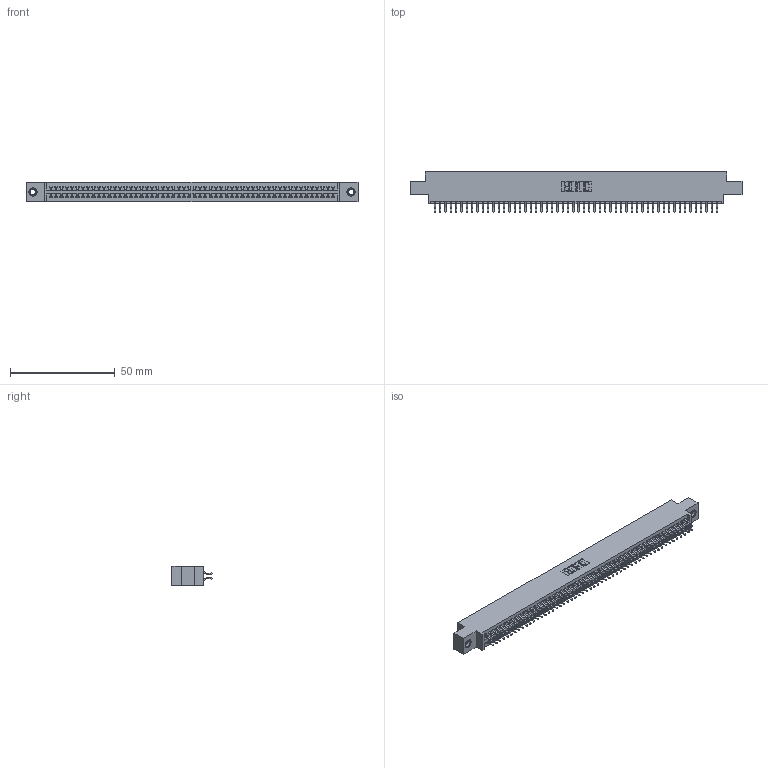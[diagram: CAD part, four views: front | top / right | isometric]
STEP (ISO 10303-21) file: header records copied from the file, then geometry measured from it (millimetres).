
FILE_DESCRIPTION (( 'STEP AP203' ), '1' );
FILE_NAME ('395-108-556-807.STEP', '2018-11-30T23:44:00', ( '' ), ( '' ), 'SwSTEP 2.0', 'SolidWorks 2016', '' );
FILE_SCHEMA (( 'CONFIG_CONTROL_DESIGN' ));
Length unit declared in the file: inch
Products named in the file (4): 395-108-556-807; 345 Part_0.170 Offset - 0.156 Dia-TI; 345-292-001_556 Tail; 345-250-001_345-250-005-103
Assembly tree (111 placements, depth 2):
  395-108-556-807
    345 Part_0.170 Offset - 0.156 Dia-TI
    345-292-001_556 Tail  x108
    345-250-001_345-250-005-103  x2
Bounding box: 158.37 x 19.24 x 9.4 mm (x, y, z)
Volume: 15364.3 mm3; surface area: 23020.3 mm2
Topology: 111 solids, 111 shells, 6238 faces, 18525 edges, 12198 vertices
Faces by surface type: plane 4112, cylinder 2110, cone 12, torus 4
Entity records: 42292 total; most frequent: CARTESIAN_POINT 7075, ORIENTED_EDGE 6990, DIRECTION 6237, EDGE_CURVE 3495, VECTOR 3119, LINE 3119, VERTEX_POINT 2324, AXIS2_PLACEMENT_3D 1559
